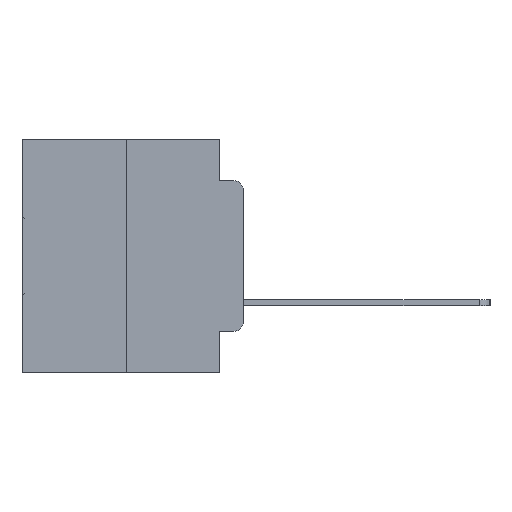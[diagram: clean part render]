
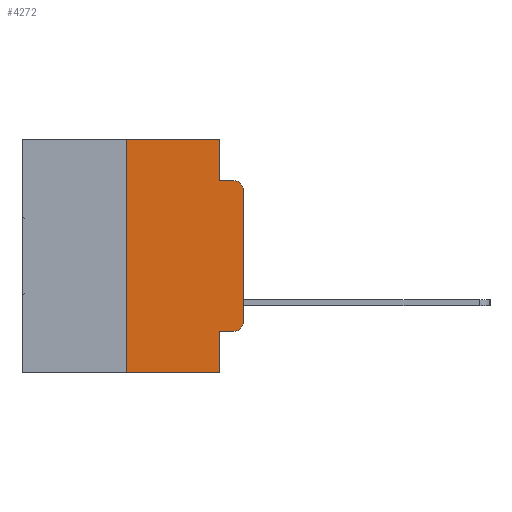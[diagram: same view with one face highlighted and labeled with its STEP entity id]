
A CAD part, left-side view. The second image highlights one B-rep face of the part: STEP entity #4272.
In plain terms, the highlighted planar face has unit normal (-1, 0, 0).
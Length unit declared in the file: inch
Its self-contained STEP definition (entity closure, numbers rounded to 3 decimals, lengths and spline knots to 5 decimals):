
#213 = CARTESIAN_POINT ( 'NONE',  ( 0., 0.051, -0.0885 ) ) ;
#220 = EDGE_CURVE ( 'NONE', #6102, #14129, #12597, .T. ) ;
#260 = VECTOR ( 'NONE', #10789, 39.37008 ) ;
#499 = EDGE_CURVE ( 'NONE', #20983, #28854, #11389, .T. ) ;
#1504 = CARTESIAN_POINT ( 'NONE',  ( 0., 0.25, -0.5 ) ) ;
#2032 = DIRECTION ( 'NONE',  ( 1., 0., 0. ) ) ;
#2169 = DIRECTION ( 'NONE',  ( 0., -1., 0. ) ) ;
#2342 = DIRECTION ( 'NONE',  ( 0., 0., 1. ) ) ;
#2455 = DIRECTION ( 'NONE',  ( 0., 0., 1. ) ) ;
#2802 = DIRECTION ( 'NONE',  ( 0., -1., 0. ) ) ;
#3877 = VECTOR ( 'NONE', #2169, 39.37008 ) ;
#4190 = VECTOR ( 'NONE', #2802, 39.37008 ) ;
#4272 = ADVANCED_FACE ( 'NONE', ( #30604 ), #14681, .F. ) ;
#4989 = LINE ( 'NONE', #213, #4190 ) ;
#5455 = LINE ( 'NONE', #5907, #32065 ) ;
#5907 = CARTESIAN_POINT ( 'NONE',  ( 0., 0.473, 0. ) ) ;
#6102 = VERTEX_POINT ( 'NONE', #15908 ) ;
#6159 = CARTESIAN_POINT ( 'NONE',  ( 0., 0.02, -0.1085 ) ) ;
#6992 = ORIENTED_EDGE ( 'NONE', *, *, #499, .T. ) ;
#7031 = EDGE_CURVE ( 'NONE', #15046, #31214, #20706, .T. ) ;
#7042 = VERTEX_POINT ( 'NONE', #12401 ) ;
#8566 = VERTEX_POINT ( 'NONE', #23114 ) ;
#8626 = ORIENTED_EDGE ( 'NONE', *, *, #25939, .F. ) ;
#8730 = DIRECTION ( 'NONE',  ( 0., 0., -1. ) ) ;
#9102 = VERTEX_POINT ( 'NONE', #17723 ) ;
#9242 = DIRECTION ( 'NONE',  ( 0., 0., -1. ) ) ;
#9872 = CARTESIAN_POINT ( 'NONE',  ( 0., 0.051, -0.4115 ) ) ;
#10146 = ORIENTED_EDGE ( 'NONE', *, *, #220, .T. ) ;
#10298 = ORIENTED_EDGE ( 'NONE', *, *, #26223, .F. ) ;
#10769 = LINE ( 'NONE', #14992, #16684 ) ;
#10789 = DIRECTION ( 'NONE',  ( 0., 0., -1. ) ) ;
#11089 = EDGE_CURVE ( 'NONE', #31214, #9102, #28655, .T. ) ;
#11389 = LINE ( 'NONE', #17310, #3877 ) ;
#11780 = ORIENTED_EDGE ( 'NONE', *, *, #17911, .F. ) ;
#12108 = CARTESIAN_POINT ( 'NONE',  ( 0., 0.473, 0. ) ) ;
#12182 = EDGE_LOOP ( 'NONE', ( #24896, #10146, #10298, #11780, #13789, #14119, #6992, #8626, #21063, #19463 ) ) ;
#12401 = CARTESIAN_POINT ( 'NONE',  ( 0., 0.051, -0.0885 ) ) ;
#12596 = CARTESIAN_POINT ( 'NONE',  ( 0., 0.02, -0.3915 ) ) ;
#12597 = CIRCLE ( 'NONE', #18423, 0.02 ) ;
#13789 = ORIENTED_EDGE ( 'NONE', *, *, #17950, .F. ) ;
#14119 = ORIENTED_EDGE ( 'NONE', *, *, #21945, .F. ) ;
#14129 = VERTEX_POINT ( 'NONE', #21805 ) ;
#14681 = PLANE ( 'NONE',  #20854 ) ;
#14992 = CARTESIAN_POINT ( 'NONE',  ( 0., 0.25, 0. ) ) ;
#15046 = VERTEX_POINT ( 'NONE', #25457 ) ;
#15161 = DIRECTION ( 'NONE',  ( 0., 0., -1. ) ) ;
#15908 = CARTESIAN_POINT ( 'NONE',  ( 0., 0., -0.1085 ) ) ;
#16684 = VECTOR ( 'NONE', #2342, 39.37008 ) ;
#17310 = CARTESIAN_POINT ( 'NONE',  ( 0., 0.473, -0.5 ) ) ;
#17587 = CARTESIAN_POINT ( 'NONE',  ( 0., 0., 0. ) ) ;
#17723 = CARTESIAN_POINT ( 'NONE',  ( 0., 0., -0.3915 ) ) ;
#17911 = EDGE_CURVE ( 'NONE', #26408, #7042, #26266, .T. ) ;
#17950 = EDGE_CURVE ( 'NONE', #8566, #26408, #5455, .T. ) ;
#18028 = VECTOR ( 'NONE', #2455, 39.37008 ) ;
#18372 = EDGE_CURVE ( 'NONE', #9102, #6102, #31256, .T. ) ;
#18423 = AXIS2_PLACEMENT_3D ( 'NONE', #6159, #23755, #8730 ) ;
#18549 = CARTESIAN_POINT ( 'NONE',  ( 0., 0.051, 0. ) ) ;
#19463 = ORIENTED_EDGE ( 'NONE', *, *, #11089, .T. ) ;
#19666 = DIRECTION ( 'NONE',  ( 0., 0., -1. ) ) ;
#20363 = LINE ( 'NONE', #26756, #26218 ) ;
#20706 = LINE ( 'NONE', #9872, #27311 ) ;
#20854 = AXIS2_PLACEMENT_3D ( 'NONE', #12108, #2032, #19666 ) ;
#20983 = VERTEX_POINT ( 'NONE', #1504 ) ;
#21063 = ORIENTED_EDGE ( 'NONE', *, *, #7031, .T. ) ;
#21606 = AXIS2_PLACEMENT_3D ( 'NONE', #12596, #30056, #15161 ) ;
#21805 = CARTESIAN_POINT ( 'NONE',  ( 0., 0.02, -0.0885 ) ) ;
#21945 = EDGE_CURVE ( 'NONE', #20983, #8566, #10769, .T. ) ;
#23114 = CARTESIAN_POINT ( 'NONE',  ( 0., 0.25, 0. ) ) ;
#23512 = DIRECTION ( 'NONE',  ( 0., -1., 0. ) ) ;
#23755 = DIRECTION ( 'NONE',  ( -1., 0., 0. ) ) ;
#24896 = ORIENTED_EDGE ( 'NONE', *, *, #18372, .T. ) ;
#25457 = CARTESIAN_POINT ( 'NONE',  ( 0., 0.051, -0.4115 ) ) ;
#25799 = CARTESIAN_POINT ( 'NONE',  ( 0., 0.051, 0. ) ) ;
#25939 = EDGE_CURVE ( 'NONE', #15046, #28854, #20363, .T. ) ;
#26218 = VECTOR ( 'NONE', #9242, 39.37008 ) ;
#26223 = EDGE_CURVE ( 'NONE', #7042, #14129, #4989, .T. ) ;
#26266 = LINE ( 'NONE', #25799, #260 ) ;
#26408 = VERTEX_POINT ( 'NONE', #18549 ) ;
#26756 = CARTESIAN_POINT ( 'NONE',  ( 0., 0.051, 0. ) ) ;
#27311 = VECTOR ( 'NONE', #27369, 39.37008 ) ;
#27369 = DIRECTION ( 'NONE',  ( 0., -1., 0. ) ) ;
#28655 = CIRCLE ( 'NONE', #21606, 0.02 ) ;
#28854 = VERTEX_POINT ( 'NONE', #29406 ) ;
#29406 = CARTESIAN_POINT ( 'NONE',  ( 0., 0.051, -0.5 ) ) ;
#30052 = CARTESIAN_POINT ( 'NONE',  ( 0., 0.02, -0.4115 ) ) ;
#30056 = DIRECTION ( 'NONE',  ( -1., 0., 0. ) ) ;
#30604 = FACE_OUTER_BOUND ( 'NONE', #12182, .T. ) ;
#31214 = VERTEX_POINT ( 'NONE', #30052 ) ;
#31256 = LINE ( 'NONE', #17587, #18028 ) ;
#32065 = VECTOR ( 'NONE', #23512, 39.37008 ) ;
